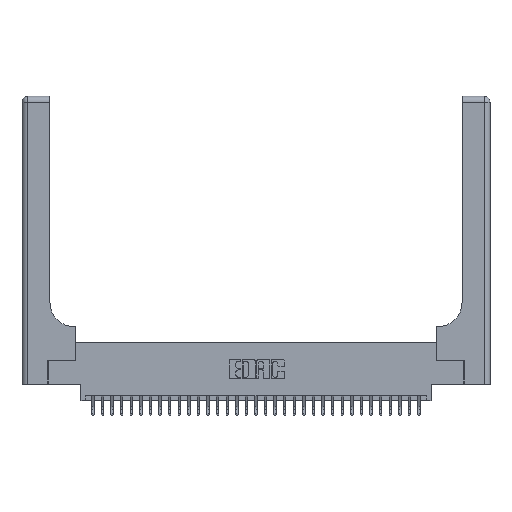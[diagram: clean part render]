
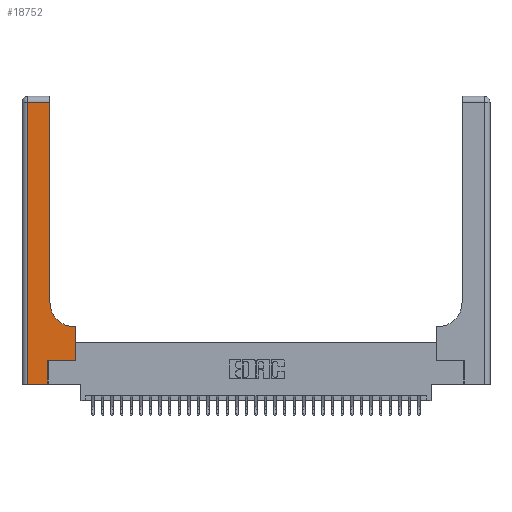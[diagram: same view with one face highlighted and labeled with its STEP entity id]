
A CAD part, top view. The second image highlights one B-rep face of the part: STEP entity #18752.
In plain terms, the highlighted planar face has unit normal (0, 0, 1).
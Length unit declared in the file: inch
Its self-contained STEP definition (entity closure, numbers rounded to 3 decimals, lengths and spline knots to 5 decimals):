
#249 = VECTOR ( 'NONE', #23833, 39.37008 ) ;
#1106 = DIRECTION ( 'NONE',  ( 1., 0., 0. ) ) ;
#1363 = CARTESIAN_POINT ( 'NONE',  ( 0.269, 0.25, 0.37 ) ) ;
#1551 = VERTEX_POINT ( 'NONE', #20655 ) ;
#1631 = CARTESIAN_POINT ( 'NONE',  ( 0.06, 2.94, 0.37 ) ) ;
#2073 = DIRECTION ( 'NONE',  ( 0., 1., 0. ) ) ;
#3386 = CARTESIAN_POINT ( 'NONE',  ( 0.269, 0.25, 0.37 ) ) ;
#3741 = EDGE_CURVE ( 'NONE', #7404, #13115, #31848, .T. ) ;
#3889 = EDGE_CURVE ( 'NONE', #13490, #23728, #11314, .T. ) ;
#4363 = DIRECTION ( 'NONE',  ( 0., 1., 0. ) ) ;
#4523 = LINE ( 'NONE', #3386, #31621 ) ;
#5058 = DIRECTION ( 'NONE',  ( 1., 0., 0. ) ) ;
#6032 = EDGE_CURVE ( 'NONE', #9835, #12106, #25047, .T. ) ;
#6711 = AXIS2_PLACEMENT_3D ( 'NONE', #13828, #16812, #6846 ) ;
#6846 = DIRECTION ( 'NONE',  ( -1., 0., 0. ) ) ;
#7404 = VERTEX_POINT ( 'NONE', #1631 ) ;
#9469 = ORIENTED_EDGE ( 'NONE', *, *, #6032, .T. ) ;
#9835 = VERTEX_POINT ( 'NONE', #30791 ) ;
#10481 = FACE_OUTER_BOUND ( 'NONE', #24787, .T. ) ;
#10694 = CARTESIAN_POINT ( 'NONE',  ( 0.06, 3., 0.37 ) ) ;
#10890 = VERTEX_POINT ( 'NONE', #1363 ) ;
#11041 = CARTESIAN_POINT ( 'NONE',  ( 0.2915, 3., 0.37 ) ) ;
#11149 = VECTOR ( 'NONE', #2073, 39.37008 ) ;
#11314 = LINE ( 'NONE', #11041, #21513 ) ;
#11727 = ORIENTED_EDGE ( 'NONE', *, *, #3889, .T. ) ;
#12106 = VERTEX_POINT ( 'NONE', #22078 ) ;
#12222 = CARTESIAN_POINT ( 'NONE',  ( 0., 0., 0.37 ) ) ;
#12788 = EDGE_CURVE ( 'NONE', #13115, #1551, #15492, .T. ) ;
#12835 = DIRECTION ( 'NONE',  ( -1., 0., 0. ) ) ;
#13115 = VERTEX_POINT ( 'NONE', #24147 ) ;
#13490 = VERTEX_POINT ( 'NONE', #29378 ) ;
#13828 = CARTESIAN_POINT ( 'NONE',  ( 0., 3., 0.37 ) ) ;
#13913 = CARTESIAN_POINT ( 'NONE',  ( 0.269, 0., 0.37 ) ) ;
#14854 = LINE ( 'NONE', #23176, #29232 ) ;
#15492 = LINE ( 'NONE', #12222, #19563 ) ;
#15932 = CIRCLE ( 'NONE', #22359, 0.25 ) ;
#15981 = EDGE_CURVE ( 'NONE', #10890, #9835, #4523, .T. ) ;
#16761 = LINE ( 'NONE', #13913, #20864 ) ;
#16812 = DIRECTION ( 'NONE',  ( 0., 0., -1. ) ) ;
#16844 = ORIENTED_EDGE ( 'NONE', *, *, #12788, .T. ) ;
#17010 = CARTESIAN_POINT ( 'NONE',  ( 0.5415, 0.6, 0.37 ) ) ;
#17539 = ORIENTED_EDGE ( 'NONE', *, *, #22144, .T. ) ;
#17974 = CARTESIAN_POINT ( 'NONE',  ( 0.5585, 0.25, 0.37 ) ) ;
#18064 = DIRECTION ( 'NONE',  ( 0., 0., -1. ) ) ;
#18186 = CARTESIAN_POINT ( 'NONE',  ( 0.2915, 0.6, 0.37 ) ) ;
#18752 = ADVANCED_FACE ( 'NONE', ( #10481 ), #29549, .F. ) ;
#19563 = VECTOR ( 'NONE', #5058, 39.37008 ) ;
#20297 = DIRECTION ( 'NONE',  ( -1., 0., 0. ) ) ;
#20587 = ORIENTED_EDGE ( 'NONE', *, *, #3741, .T. ) ;
#20655 = CARTESIAN_POINT ( 'NONE',  ( 0.269, 0., 0.37 ) ) ;
#20864 = VECTOR ( 'NONE', #29290, 39.37008 ) ;
#21492 = VERTEX_POINT ( 'NONE', #17010 ) ;
#21513 = VECTOR ( 'NONE', #4363, 39.37008 ) ;
#22078 = CARTESIAN_POINT ( 'NONE',  ( 0.5585, 0.6, 0.37 ) ) ;
#22144 = EDGE_CURVE ( 'NONE', #21492, #13490, #15932, .T. ) ;
#22359 = AXIS2_PLACEMENT_3D ( 'NONE', #33696, #18064, #33922 ) ;
#23176 = CARTESIAN_POINT ( 'NONE',  ( 0., 2.94, 0.37 ) ) ;
#23545 = CARTESIAN_POINT ( 'NONE',  ( 0.2915, 2.94, 0.37 ) ) ;
#23728 = VERTEX_POINT ( 'NONE', #23545 ) ;
#23790 = LINE ( 'NONE', #18186, #28737 ) ;
#23833 = DIRECTION ( 'NONE',  ( 0., -1., 0. ) ) ;
#24147 = CARTESIAN_POINT ( 'NONE',  ( 0.06, 0., 0.37 ) ) ;
#24787 = EDGE_LOOP ( 'NONE', ( #11727, #31864, #20587, #16844, #27471, #32062, #9469, #30917, #17539 ) ) ;
#25047 = LINE ( 'NONE', #17974, #11149 ) ;
#27471 = ORIENTED_EDGE ( 'NONE', *, *, #32132, .T. ) ;
#28737 = VECTOR ( 'NONE', #12835, 39.37008 ) ;
#29232 = VECTOR ( 'NONE', #20297, 39.37008 ) ;
#29290 = DIRECTION ( 'NONE',  ( 0., 1., 0. ) ) ;
#29378 = CARTESIAN_POINT ( 'NONE',  ( 0.2915, 0.85, 0.37 ) ) ;
#29549 = PLANE ( 'NONE',  #6711 ) ;
#30352 = EDGE_CURVE ( 'NONE', #23728, #7404, #14854, .T. ) ;
#30791 = CARTESIAN_POINT ( 'NONE',  ( 0.5585, 0.25, 0.37 ) ) ;
#30917 = ORIENTED_EDGE ( 'NONE', *, *, #31215, .T. ) ;
#31215 = EDGE_CURVE ( 'NONE', #12106, #21492, #23790, .T. ) ;
#31621 = VECTOR ( 'NONE', #1106, 39.37008 ) ;
#31848 = LINE ( 'NONE', #10694, #249 ) ;
#31864 = ORIENTED_EDGE ( 'NONE', *, *, #30352, .T. ) ;
#32062 = ORIENTED_EDGE ( 'NONE', *, *, #15981, .T. ) ;
#32132 = EDGE_CURVE ( 'NONE', #1551, #10890, #16761, .T. ) ;
#33696 = CARTESIAN_POINT ( 'NONE',  ( 0.5415, 0.85, 0.37 ) ) ;
#33922 = DIRECTION ( 'NONE',  ( 1., 0., 0. ) ) ;
